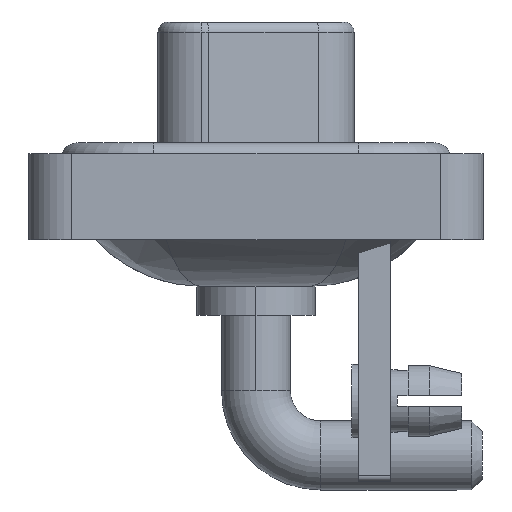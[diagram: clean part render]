
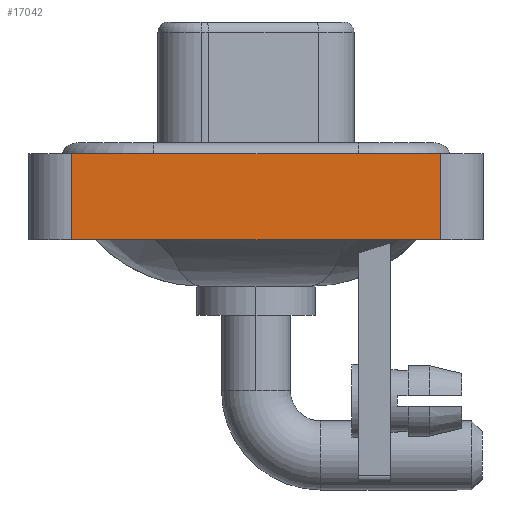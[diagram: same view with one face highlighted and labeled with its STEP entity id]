
A CAD part, left-side view. The second image highlights one B-rep face of the part: STEP entity #17042.
In plain terms, the highlighted planar face has unit normal (-1, 0, 0).
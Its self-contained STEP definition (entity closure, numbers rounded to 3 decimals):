
#58 = VECTOR ( 'NONE', #15253, 1000. ) ;
#1425 = DIRECTION ( 'NONE',  ( 0., -1., 0. ) ) ;
#1639 = AXIS2_PLACEMENT_3D ( 'NONE', #8114, #17774, #3713 ) ;
#2949 = LINE ( 'NONE', #15478, #11091 ) ;
#3713 = DIRECTION ( 'NONE',  ( 0., 0., 1. ) ) ;
#3809 = FACE_OUTER_BOUND ( 'NONE', #17049, .T. ) ;
#3963 = CARTESIAN_POINT ( 'NONE',  ( -7.25, -8.55, 0.4 ) ) ;
#4382 = DIRECTION ( 'NONE',  ( 0., 0., 1. ) ) ;
#4974 = DIRECTION ( 'NONE',  ( 0., 0., 1. ) ) ;
#7132 = LINE ( 'NONE', #3963, #58 ) ;
#7558 = LINE ( 'NONE', #19862, #14405 ) ;
#8114 = CARTESIAN_POINT ( 'NONE',  ( -7.25, -8.55, -3.6 ) ) ;
#8142 = EDGE_CURVE ( 'NONE', #13937, #12515, #2949, .T. ) ;
#8346 = EDGE_CURVE ( 'NONE', #12515, #10761, #12769, .T. ) ;
#9006 = ORIENTED_EDGE ( 'NONE', *, *, #17557, .F. ) ;
#9337 = ORIENTED_EDGE ( 'NONE', *, *, #8142, .T. ) ;
#9359 = CARTESIAN_POINT ( 'NONE',  ( -7.25, 8.55, 0.4 ) ) ;
#10761 = VERTEX_POINT ( 'NONE', #19650 ) ;
#11091 = VECTOR ( 'NONE', #1425, 1000. ) ;
#11100 = VECTOR ( 'NONE', #4974, 1000. ) ;
#12515 = VERTEX_POINT ( 'NONE', #17606 ) ;
#12732 = ORIENTED_EDGE ( 'NONE', *, *, #14996, .F. ) ;
#12769 = LINE ( 'NONE', #19032, #11100 ) ;
#13937 = VERTEX_POINT ( 'NONE', #16130 ) ;
#14405 = VECTOR ( 'NONE', #4382, 1000. ) ;
#14996 = EDGE_CURVE ( 'NONE', #20131, #10761, #7132, .T. ) ;
#15253 = DIRECTION ( 'NONE',  ( 0., -1., 0. ) ) ;
#15478 = CARTESIAN_POINT ( 'NONE',  ( -7.25, -8.55, -3.6 ) ) ;
#15726 = ORIENTED_EDGE ( 'NONE', *, *, #8346, .T. ) ;
#16130 = CARTESIAN_POINT ( 'NONE',  ( -7.25, 8.55, -3.6 ) ) ;
#17042 = ADVANCED_FACE ( 'NONE', ( #3809 ), #19306, .T. ) ;
#17049 = EDGE_LOOP ( 'NONE', ( #15726, #12732, #9006, #9337 ) ) ;
#17557 = EDGE_CURVE ( 'NONE', #13937, #20131, #7558, .T. ) ;
#17606 = CARTESIAN_POINT ( 'NONE',  ( -7.25, -8.55, -3.6 ) ) ;
#17774 = DIRECTION ( 'NONE',  ( -1., 0., 0. ) ) ;
#19032 = CARTESIAN_POINT ( 'NONE',  ( -7.25, -8.55, -3.6 ) ) ;
#19306 = PLANE ( 'NONE',  #1639 ) ;
#19650 = CARTESIAN_POINT ( 'NONE',  ( -7.25, -8.55, 0.4 ) ) ;
#19862 = CARTESIAN_POINT ( 'NONE',  ( -7.25, 8.55, -3.6 ) ) ;
#20131 = VERTEX_POINT ( 'NONE', #9359 ) ;
